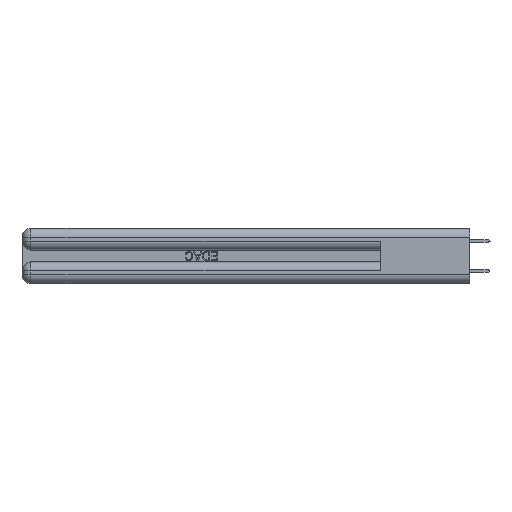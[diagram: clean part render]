
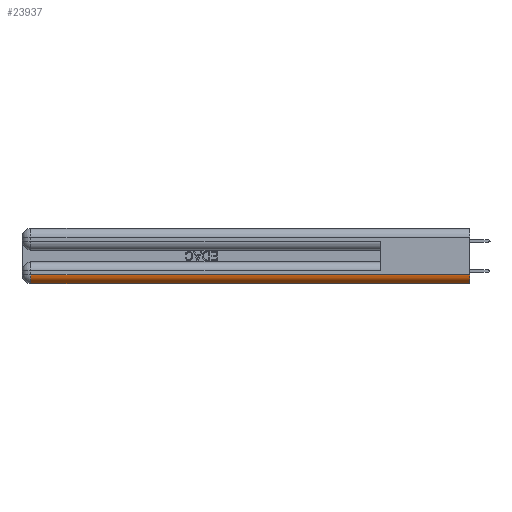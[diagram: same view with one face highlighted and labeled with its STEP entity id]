
A CAD part, left-side view. The second image highlights one B-rep face of the part: STEP entity #23937.
In plain terms, the highlighted cylindrical face has radius 1.524 mm (diameter 3.048 mm), a partial arc.
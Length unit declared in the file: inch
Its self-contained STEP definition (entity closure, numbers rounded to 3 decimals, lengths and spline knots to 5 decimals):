
#1149 = VECTOR ( 'NONE', #10496, 39.37008 ) ;
#1276 = DIRECTION ( 'NONE',  ( 0., 0., 1. ) ) ;
#1964 = ORIENTED_EDGE ( 'NONE', *, *, #10058, .F. ) ;
#2199 = DIRECTION ( 'NONE',  ( 0., 1., 0. ) ) ;
#5370 = VERTEX_POINT ( 'NONE', #29413 ) ;
#8689 = VERTEX_POINT ( 'NONE', #41537 ) ;
#9924 = DIRECTION ( 'NONE',  ( 0., -1., 0. ) ) ;
#10058 = EDGE_CURVE ( 'NONE', #17782, #35052, #33241, .T. ) ;
#10496 = DIRECTION ( 'NONE',  ( 0., -1., 0. ) ) ;
#10576 = ORIENTED_EDGE ( 'NONE', *, *, #40114, .F. ) ;
#13989 = FACE_OUTER_BOUND ( 'NONE', #24391, .T. ) ;
#14112 = DIRECTION ( 'NONE',  ( 0., 0., 1. ) ) ;
#14637 = AXIS2_PLACEMENT_3D ( 'NONE', #36830, #33712, #1276 ) ;
#15130 = EDGE_CURVE ( 'NONE', #8689, #17782, #42488, .T. ) ;
#17659 = DIRECTION ( 'NONE',  ( 0., 1., 0. ) ) ;
#17782 = VERTEX_POINT ( 'NONE', #45932 ) ;
#19038 = CARTESIAN_POINT ( 'NONE',  ( 0.06, 2.94, 0.06 ) ) ;
#19843 = AXIS2_PLACEMENT_3D ( 'NONE', #19038, #2199, #14112 ) ;
#21255 = CYLINDRICAL_SURFACE ( 'NONE', #14637, 0.06 ) ;
#22934 = CARTESIAN_POINT ( 'NONE',  ( 0., 0., 0.06 ) ) ;
#23937 = ADVANCED_FACE ( 'NONE', ( #13989 ), #21255, .T. ) ;
#24391 = EDGE_LOOP ( 'NONE', ( #32213, #10576, #46087, #1964 ) ) ;
#26420 = CIRCLE ( 'NONE', #19843, 0.06 ) ;
#26817 = CARTESIAN_POINT ( 'NONE',  ( 0.06, 2.94, 0. ) ) ;
#29413 = CARTESIAN_POINT ( 'NONE',  ( 0., 2.94, 0.06 ) ) ;
#29897 = DIRECTION ( 'NONE',  ( 0., 0., 1. ) ) ;
#31722 = AXIS2_PLACEMENT_3D ( 'NONE', #41340, #9924, #29897 ) ;
#31846 = VECTOR ( 'NONE', #17659, 39.37008 ) ;
#32213 = ORIENTED_EDGE ( 'NONE', *, *, #15130, .F. ) ;
#33241 = LINE ( 'NONE', #49553, #31846 ) ;
#33712 = DIRECTION ( 'NONE',  ( 0., 1., 0. ) ) ;
#35052 = VERTEX_POINT ( 'NONE', #26817 ) ;
#36830 = CARTESIAN_POINT ( 'NONE',  ( 0.06, 0., 0.06 ) ) ;
#40114 = EDGE_CURVE ( 'NONE', #5370, #8689, #50664, .T. ) ;
#41340 = CARTESIAN_POINT ( 'NONE',  ( 0.06, 0., 0.06 ) ) ;
#41537 = CARTESIAN_POINT ( 'NONE',  ( 0., 0., 0.06 ) ) ;
#42488 = CIRCLE ( 'NONE', #31722, 0.06 ) ;
#45932 = CARTESIAN_POINT ( 'NONE',  ( 0.06, 0., 0. ) ) ;
#46087 = ORIENTED_EDGE ( 'NONE', *, *, #48134, .F. ) ;
#48134 = EDGE_CURVE ( 'NONE', #35052, #5370, #26420, .T. ) ;
#49553 = CARTESIAN_POINT ( 'NONE',  ( 0.06, 3., 0. ) ) ;
#50664 = LINE ( 'NONE', #22934, #1149 ) ;
